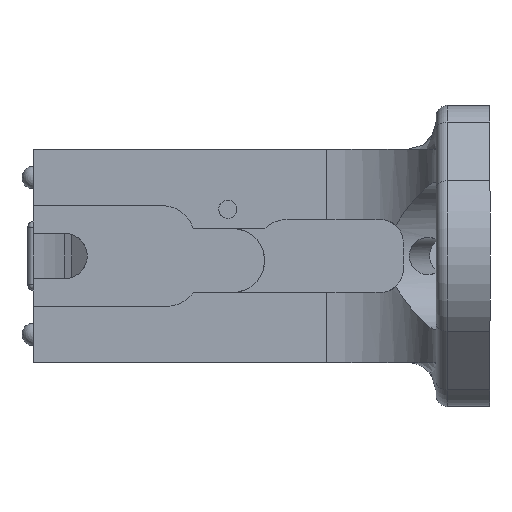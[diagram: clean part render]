
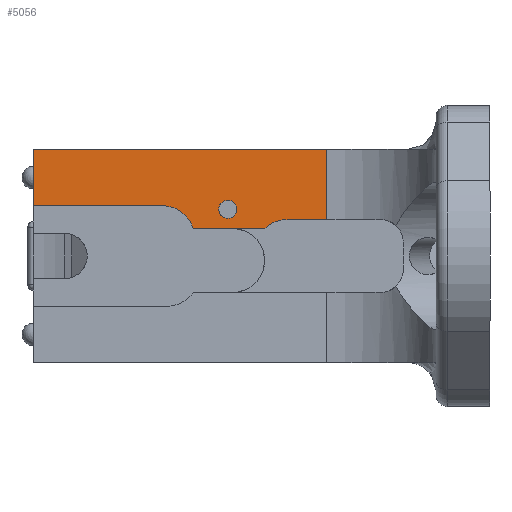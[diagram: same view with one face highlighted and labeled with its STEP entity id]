
A CAD part, left-side view. The second image highlights one B-rep face of the part: STEP entity #5056.
In plain terms, the highlighted planar face has unit normal (-1, 0, 0).
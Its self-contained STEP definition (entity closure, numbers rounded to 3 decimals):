
#78 = VERTEX_POINT ( 'NONE', #6867 ) ;
#596 = LINE ( 'NONE', #3639, #9409 ) ;
#643 = ORIENTED_EDGE ( 'NONE', *, *, #7246, .T. ) ;
#649 = FACE_BOUND ( 'NONE', #8737, .T. ) ;
#699 = VERTEX_POINT ( 'NONE', #7824 ) ;
#828 = CARTESIAN_POINT ( 'NONE',  ( -90.919, 66.528, -855.789 ) ) ;
#861 = CIRCLE ( 'NONE', #2830, 1.587 ) ;
#888 = PLANE ( 'NONE',  #4025 ) ;
#1340 = EDGE_CURVE ( 'NONE', #699, #9697, #8008, .T. ) ;
#1623 = ORIENTED_EDGE ( 'NONE', *, *, #8778, .T. ) ;
#1773 = CARTESIAN_POINT ( 'NONE',  ( -90.919, 174.168, -9.74 ) ) ;
#2087 = ORIENTED_EDGE ( 'NONE', *, *, #9443, .T. ) ;
#2677 = CARTESIAN_POINT ( 'NONE',  ( -90.919, 32.64, 12.683 ) ) ;
#2684 = AXIS2_PLACEMENT_3D ( 'NONE', #4755, #10864, #5643 ) ;
#2830 = AXIS2_PLACEMENT_3D ( 'NONE', #2677, #8836, #3571 ) ;
#2854 = CARTESIAN_POINT ( 'NONE',  ( -90.919, 22.338, 5.341 ) ) ;
#3007 = FACE_OUTER_BOUND ( 'NONE', #10319, .T. ) ;
#3115 = LINE ( 'NONE', #10192, #5769 ) ;
#3312 = VECTOR ( 'NONE', #5034, 1000. ) ;
#3322 = DIRECTION ( 'NONE',  ( 0., 0., 1. ) ) ;
#3363 = ORIENTED_EDGE ( 'NONE', *, *, #9009, .T. ) ;
#3571 = DIRECTION ( 'NONE',  ( 0., 0., -1. ) ) ;
#3610 = DIRECTION ( 'NONE',  ( 0., -1., 0. ) ) ;
#3639 = CARTESIAN_POINT ( 'NONE',  ( -90.919, 225.699, 23.114 ) ) ;
#3746 = CARTESIAN_POINT ( 'NONE',  ( -90.919, 44.015, 13.31 ) ) ;
#3756 = DIRECTION ( 'NONE',  ( 0., -1., 0. ) ) ;
#3916 = LINE ( 'NONE', #6817, #8578 ) ;
#3936 = ORIENTED_EDGE ( 'NONE', *, *, #4950, .T. ) ;
#4025 = AXIS2_PLACEMENT_3D ( 'NONE', #1773, #8865, #3610 ) ;
#4159 = CARTESIAN_POINT ( 'NONE',  ( -90.919, 174.168, 9.323 ) ) ;
#4345 = EDGE_CURVE ( 'NONE', #7507, #699, #5123, .T. ) ;
#4540 = VERTEX_POINT ( 'NONE', #6207 ) ;
#4570 = AXIS2_PLACEMENT_3D ( 'NONE', #2854, #9013, #3756 ) ;
#4755 = CARTESIAN_POINT ( 'NONE',  ( -90.919, 44.015, 7.754 ) ) ;
#4950 = EDGE_CURVE ( 'NONE', #4540, #78, #10299, .T. ) ;
#4960 = DIRECTION ( 'NONE',  ( 0., -1., 0. ) ) ;
#5034 = DIRECTION ( 'NONE',  ( 0., -1., 0. ) ) ;
#5056 = ADVANCED_FACE ( 'NONE', ( #649, #3007 ), #888, .T. ) ;
#5123 = CIRCLE ( 'NONE', #2684, 5.556 ) ;
#5569 = ORIENTED_EDGE ( 'NONE', *, *, #9753, .T. ) ;
#5643 = DIRECTION ( 'NONE',  ( 0., -1., 0. ) ) ;
#5769 = VECTOR ( 'NONE', #4960, 1000. ) ;
#5926 = DIRECTION ( 'NONE',  ( 0., -1., 0. ) ) ;
#6207 = CARTESIAN_POINT ( 'NONE',  ( -90.919, 15.418, 10.897 ) ) ;
#6401 = VERTEX_POINT ( 'NONE', #11291 ) ;
#6533 = VERTEX_POINT ( 'NONE', #7336 ) ;
#6617 = CARTESIAN_POINT ( 'NONE',  ( -90.919, 26.213, 9.323 ) ) ;
#6817 = CARTESIAN_POINT ( 'NONE',  ( -90.919, 174.168, 10.897 ) ) ;
#6867 = CARTESIAN_POINT ( 'NONE',  ( -90.919, 15.418, 23.114 ) ) ;
#6922 = ORIENTED_EDGE ( 'NONE', *, *, #8688, .T. ) ;
#7246 = EDGE_CURVE ( 'NONE', #6401, #7507, #3115, .T. ) ;
#7336 = CARTESIAN_POINT ( 'NONE',  ( -90.919, 66.528, 23.114 ) ) ;
#7507 = VERTEX_POINT ( 'NONE', #3746 ) ;
#7674 = CARTESIAN_POINT ( 'NONE',  ( -90.919, 22.338, 10.897 ) ) ;
#7731 = ORIENTED_EDGE ( 'NONE', *, *, #4345, .T. ) ;
#7824 = CARTESIAN_POINT ( 'NONE',  ( -90.919, 38.685, 9.323 ) ) ;
#7977 = VECTOR ( 'NONE', #3322, 1000. ) ;
#8008 = LINE ( 'NONE', #4159, #3312 ) ;
#8288 = CARTESIAN_POINT ( 'NONE',  ( -90.919, 32.64, 11.096 ) ) ;
#8578 = VECTOR ( 'NONE', #5926, 1000. ) ;
#8598 = CARTESIAN_POINT ( 'NONE',  ( -90.919, 15.418, -13.919 ) ) ;
#8688 = EDGE_CURVE ( 'NONE', #78, #6533, #596, .T. ) ;
#8737 = EDGE_LOOP ( 'NONE', ( #2087 ) ) ;
#8777 = DIRECTION ( 'NONE',  ( 0., 1., 0. ) ) ;
#8778 = EDGE_CURVE ( 'NONE', #9697, #10360, #11181, .T. ) ;
#8836 = DIRECTION ( 'NONE',  ( 1., 0., 0. ) ) ;
#8865 = DIRECTION ( 'NONE',  ( -1., 0., 0. ) ) ;
#9009 = EDGE_CURVE ( 'NONE', #6533, #6401, #10094, .T. ) ;
#9013 = DIRECTION ( 'NONE',  ( 1., 0., 0. ) ) ;
#9409 = VECTOR ( 'NONE', #8777, 1000. ) ;
#9443 = EDGE_CURVE ( 'NONE', #11007, #11007, #861, .T. ) ;
#9697 = VERTEX_POINT ( 'NONE', #6617 ) ;
#9753 = EDGE_CURVE ( 'NONE', #10360, #4540, #3916, .T. ) ;
#9830 = VECTOR ( 'NONE', #10488, 1000. ) ;
#10094 = LINE ( 'NONE', #828, #9830 ) ;
#10192 = CARTESIAN_POINT ( 'NONE',  ( -90.919, 174.168, 13.31 ) ) ;
#10299 = LINE ( 'NONE', #8598, #7977 ) ;
#10319 = EDGE_LOOP ( 'NONE', ( #3936, #6922, #3363, #643, #7731, #11340, #1623, #5569 ) ) ;
#10360 = VERTEX_POINT ( 'NONE', #7674 ) ;
#10488 = DIRECTION ( 'NONE',  ( 0., 0., -1. ) ) ;
#10864 = DIRECTION ( 'NONE',  ( 1., 0., 0. ) ) ;
#11007 = VERTEX_POINT ( 'NONE', #8288 ) ;
#11181 = CIRCLE ( 'NONE', #4570, 5.556 ) ;
#11291 = CARTESIAN_POINT ( 'NONE',  ( -90.919, 66.528, 13.31 ) ) ;
#11340 = ORIENTED_EDGE ( 'NONE', *, *, #1340, .T. ) ;
